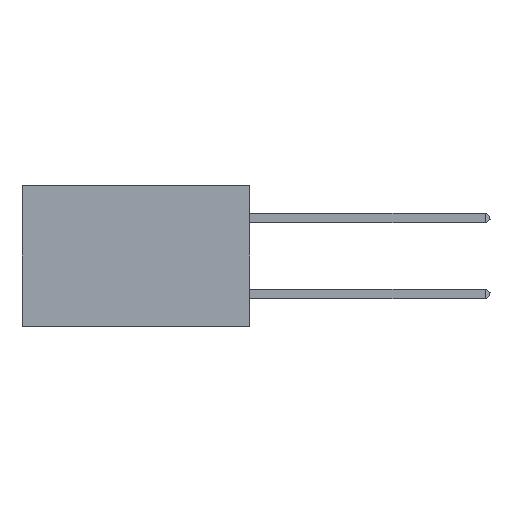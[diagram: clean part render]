
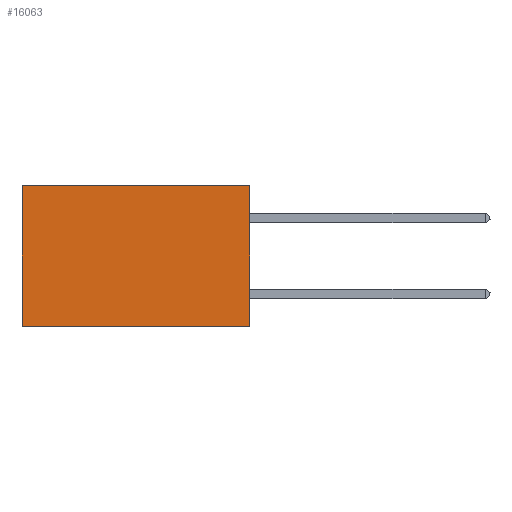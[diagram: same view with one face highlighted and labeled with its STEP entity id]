
A CAD part, left-side view. The second image highlights one B-rep face of the part: STEP entity #16063.
In plain terms, the highlighted planar face has unit normal (-1, 0, 0).
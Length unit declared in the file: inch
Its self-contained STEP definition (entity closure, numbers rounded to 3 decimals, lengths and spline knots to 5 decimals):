
#174 = DIRECTION ( 'NONE',  ( 0., 0., -1. ) ) ;
#727 = VECTOR ( 'NONE', #45007, 39.37008 ) ;
#1511 = ORIENTED_EDGE ( 'NONE', *, *, #32605, .F. ) ;
#1578 = DIRECTION ( 'NONE',  ( 0., 0., -1. ) ) ;
#3342 = LINE ( 'NONE', #9871, #30310 ) ;
#6562 = DIRECTION ( 'NONE',  ( 0., 1., 0. ) ) ;
#7182 = EDGE_CURVE ( 'NONE', #24275, #21903, #3342, .T. ) ;
#8175 = ORIENTED_EDGE ( 'NONE', *, *, #22822, .T. ) ;
#9871 = CARTESIAN_POINT ( 'NONE',  ( 0.2875, 0., -0.37 ) ) ;
#10159 = FACE_OUTER_BOUND ( 'NONE', #34710, .T. ) ;
#10751 = CARTESIAN_POINT ( 'NONE',  ( 0.2875, 0.6, 0. ) ) ;
#13601 = CARTESIAN_POINT ( 'NONE',  ( 0.2875, 0., 0. ) ) ;
#14951 = VERTEX_POINT ( 'NONE', #16978 ) ;
#15630 = DIRECTION ( 'NONE',  ( 1., 0., 0. ) ) ;
#15805 = LINE ( 'NONE', #19887, #727 ) ;
#16063 = ADVANCED_FACE ( 'NONE', ( #10159 ), #18922, .F. ) ;
#16978 = CARTESIAN_POINT ( 'NONE',  ( 0.2875, 0., 0. ) ) ;
#18336 = EDGE_CURVE ( 'NONE', #39797, #21903, #35855, .T. ) ;
#18922 = PLANE ( 'NONE',  #26195 ) ;
#19075 = CARTESIAN_POINT ( 'NONE',  ( 0.2875, 0., 0. ) ) ;
#19887 = CARTESIAN_POINT ( 'NONE',  ( 0.2875, 0., 0. ) ) ;
#21903 = VERTEX_POINT ( 'NONE', #26504 ) ;
#22822 = EDGE_CURVE ( 'NONE', #14951, #39797, #33251, .T. ) ;
#24275 = VERTEX_POINT ( 'NONE', #26750 ) ;
#26195 = AXIS2_PLACEMENT_3D ( 'NONE', #19075, #15630, #1578 ) ;
#26504 = CARTESIAN_POINT ( 'NONE',  ( 0.2875, 0.6, -0.37 ) ) ;
#26750 = CARTESIAN_POINT ( 'NONE',  ( 0.2875, 0., -0.37 ) ) ;
#29287 = VECTOR ( 'NONE', #6562, 39.37008 ) ;
#30310 = VECTOR ( 'NONE', #30924, 39.37008 ) ;
#30646 = CARTESIAN_POINT ( 'NONE',  ( 0.2875, 0.6, 0. ) ) ;
#30924 = DIRECTION ( 'NONE',  ( 0., 1., 0. ) ) ;
#32605 = EDGE_CURVE ( 'NONE', #14951, #24275, #15805, .T. ) ;
#33251 = LINE ( 'NONE', #13601, #29287 ) ;
#34710 = EDGE_LOOP ( 'NONE', ( #35215, #41890, #1511, #8175 ) ) ;
#35215 = ORIENTED_EDGE ( 'NONE', *, *, #18336, .T. ) ;
#35855 = LINE ( 'NONE', #10751, #39750 ) ;
#39750 = VECTOR ( 'NONE', #174, 39.37008 ) ;
#39797 = VERTEX_POINT ( 'NONE', #30646 ) ;
#41890 = ORIENTED_EDGE ( 'NONE', *, *, #7182, .F. ) ;
#45007 = DIRECTION ( 'NONE',  ( 0., 0., -1. ) ) ;
